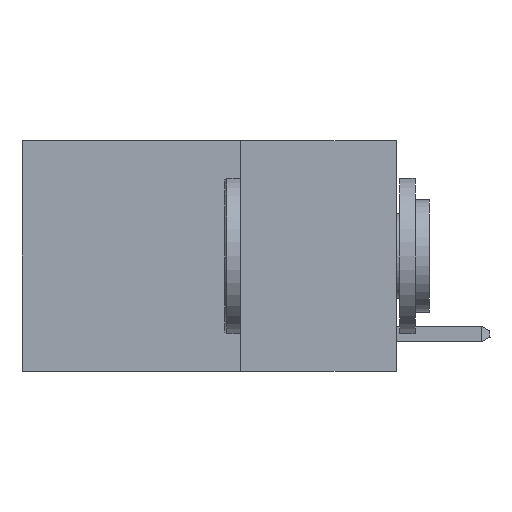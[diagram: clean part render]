
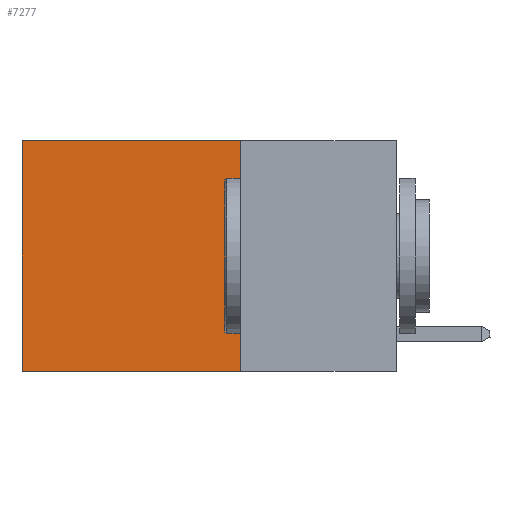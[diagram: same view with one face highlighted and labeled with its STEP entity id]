
A CAD part, left-side view. The second image highlights one B-rep face of the part: STEP entity #7277.
In plain terms, the highlighted planar face has unit normal (-1, 0, 0).
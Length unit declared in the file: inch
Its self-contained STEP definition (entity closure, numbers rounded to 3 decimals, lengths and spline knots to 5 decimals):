
#464 = LINE ( 'NONE', #11991, #9662 ) ;
#1209 = ORIENTED_EDGE ( 'NONE', *, *, #3213, .T. ) ;
#1435 = EDGE_CURVE ( 'NONE', #8499, #9001, #464, .T. ) ;
#1687 = AXIS2_PLACEMENT_3D ( 'NONE', #3710, #5628, #10354 ) ;
#1704 = ORIENTED_EDGE ( 'NONE', *, *, #2843, .T. ) ;
#2442 = CARTESIAN_POINT ( 'NONE',  ( 0.2625, 0.25, -0.37 ) ) ;
#2843 = EDGE_CURVE ( 'NONE', #9265, #9001, #7537, .T. ) ;
#3213 = EDGE_CURVE ( 'NONE', #10183, #9265, #12103, .T. ) ;
#3361 = CARTESIAN_POINT ( 'NONE',  ( 0.2625, 0.25, 0. ) ) ;
#3442 = CARTESIAN_POINT ( 'NONE',  ( 0.2625, 0.25, 0. ) ) ;
#3710 = CARTESIAN_POINT ( 'NONE',  ( 0.2625, 0.25, 0. ) ) ;
#4132 = ORIENTED_EDGE ( 'NONE', *, *, #8466, .F. ) ;
#4345 = DIRECTION ( 'NONE',  ( 0., 1., 0. ) ) ;
#4488 = FACE_OUTER_BOUND ( 'NONE', #7867, .T. ) ;
#4778 = CARTESIAN_POINT ( 'NONE',  ( 0.2625, 0.6, -0.37 ) ) ;
#5628 = DIRECTION ( 'NONE',  ( 1., 0., 0. ) ) ;
#7236 = CARTESIAN_POINT ( 'NONE',  ( 0.2625, 0.25, 0. ) ) ;
#7267 = DIRECTION ( 'NONE',  ( 0., 1., 0. ) ) ;
#7277 = ADVANCED_FACE ( 'NONE', ( #4488 ), #12263, .F. ) ;
#7499 = VECTOR ( 'NONE', #11124, 39.37008 ) ;
#7537 = LINE ( 'NONE', #9638, #10736 ) ;
#7867 = EDGE_LOOP ( 'NONE', ( #1704, #10795, #4132, #1209 ) ) ;
#8463 = DIRECTION ( 'NONE',  ( 0., 0., -1. ) ) ;
#8466 = EDGE_CURVE ( 'NONE', #10183, #8499, #10043, .T. ) ;
#8499 = VERTEX_POINT ( 'NONE', #2442 ) ;
#9001 = VERTEX_POINT ( 'NONE', #4778 ) ;
#9265 = VERTEX_POINT ( 'NONE', #10075 ) ;
#9638 = CARTESIAN_POINT ( 'NONE',  ( 0.2625, 0.6, 0. ) ) ;
#9662 = VECTOR ( 'NONE', #4345, 39.37008 ) ;
#10043 = LINE ( 'NONE', #7236, #7499 ) ;
#10075 = CARTESIAN_POINT ( 'NONE',  ( 0.2625, 0.6, 0. ) ) ;
#10183 = VERTEX_POINT ( 'NONE', #3442 ) ;
#10354 = DIRECTION ( 'NONE',  ( 0., 0., -1. ) ) ;
#10736 = VECTOR ( 'NONE', #8463, 39.37008 ) ;
#10795 = ORIENTED_EDGE ( 'NONE', *, *, #1435, .F. ) ;
#11124 = DIRECTION ( 'NONE',  ( 0., 0., -1. ) ) ;
#11991 = CARTESIAN_POINT ( 'NONE',  ( 0.2625, 0.25, -0.37 ) ) ;
#12103 = LINE ( 'NONE', #3361, #12378 ) ;
#12263 = PLANE ( 'NONE',  #1687 ) ;
#12378 = VECTOR ( 'NONE', #7267, 39.37008 ) ;
